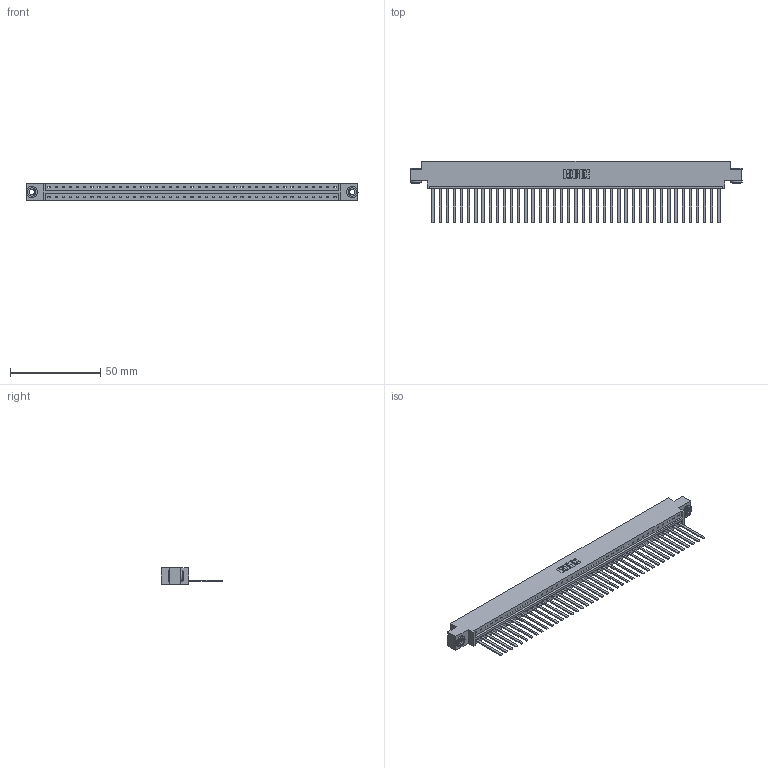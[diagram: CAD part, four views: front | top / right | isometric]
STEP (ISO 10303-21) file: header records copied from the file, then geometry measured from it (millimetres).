
FILE_DESCRIPTION (( 'STEP AP203' ), '1' );
FILE_NAME ('833-041-544-603.STEP', '2020-06-03T19:33:26', ( '' ), ( '' ), 'SwSTEP 2.0', 'SolidWorks 2020', '' );
FILE_SCHEMA (( 'CONFIG_CONTROL_DESIGN' ));
Length unit declared in the file: inch
Products named in the file (4): 345-292-001_345-293-144; 833-041-544-603; 345-250-002_345-250-002-102; 833 Part_Offset - .156 Dia - TH
Assembly tree (44 placements, depth 2):
  833-041-544-603
    833 Part_Offset - .156 Dia - TH
    345-292-001_345-293-144  x41
    345-250-002_345-250-002-102  x2
Bounding box: 184 x 34.3 x 9.4 mm (x, y, z)
Volume: 18773.2 mm3; surface area: 22275.3 mm2
Topology: 44 solids, 44 shells, 2288 faces, 6877 edges, 4526 vertices
Faces by surface type: plane 1642, cylinder 638, cone 8
Entity records: 25792 total; most frequent: CARTESIAN_POINT 4428, ORIENTED_EDGE 4398, DIRECTION 3767, EDGE_CURVE 2199, LINE 2051, VECTOR 2051, VERTEX_POINT 1462, AXIS2_PLACEMENT_3D 858
